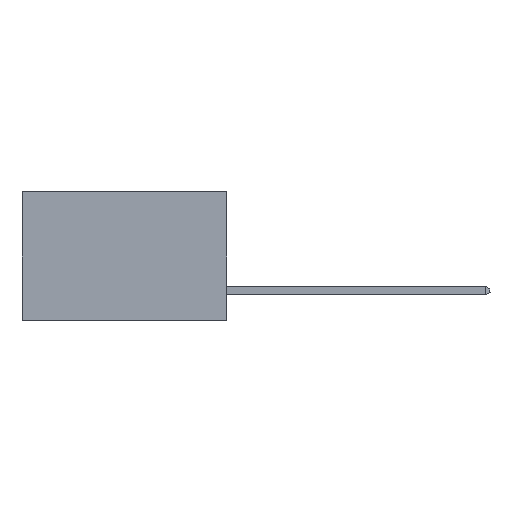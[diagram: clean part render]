
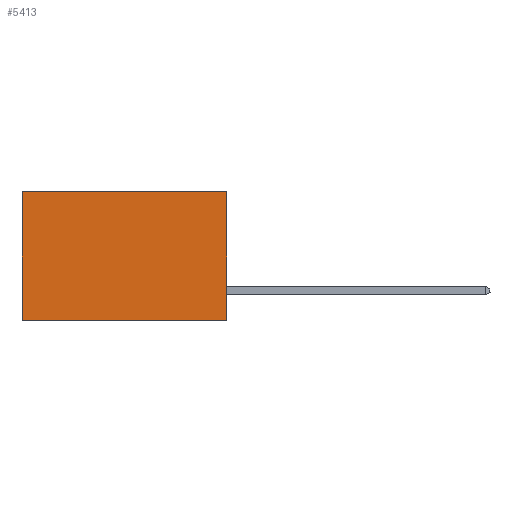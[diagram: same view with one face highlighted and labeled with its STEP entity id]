
A CAD part, left-side view. The second image highlights one B-rep face of the part: STEP entity #5413.
In plain terms, the highlighted planar face has unit normal (-1, 0, 0).
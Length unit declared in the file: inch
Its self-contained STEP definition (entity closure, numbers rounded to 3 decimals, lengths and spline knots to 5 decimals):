
#624 = ORIENTED_EDGE ( 'NONE', *, *, #3565, .F. ) ;
#1215 = CARTESIAN_POINT ( 'NONE',  ( 0.277, 0., -0.37 ) ) ;
#1657 = EDGE_CURVE ( 'NONE', #7869, #6079, #14360, .T. ) ;
#2672 = EDGE_CURVE ( 'NONE', #15554, #18277, #18735, .T. ) ;
#3064 = AXIS2_PLACEMENT_3D ( 'NONE', #20327, #19567, #19518 ) ;
#3565 = EDGE_CURVE ( 'NONE', #6079, #18277, #11058, .T. ) ;
#3865 = LINE ( 'NONE', #8832, #11904 ) ;
#4542 = CARTESIAN_POINT ( 'NONE',  ( 0.277, 0., 0. ) ) ;
#5362 = CARTESIAN_POINT ( 'NONE',  ( 0.277, 0.59, 0. ) ) ;
#5413 = ADVANCED_FACE ( 'NONE', ( #12937 ), #20309, .F. ) ;
#6079 = VERTEX_POINT ( 'NONE', #1215 ) ;
#7869 = VERTEX_POINT ( 'NONE', #4542 ) ;
#8792 = ORIENTED_EDGE ( 'NONE', *, *, #20197, .T. ) ;
#8832 = CARTESIAN_POINT ( 'NONE',  ( 0.277, 0., 0. ) ) ;
#10455 = DIRECTION ( 'NONE',  ( 0., 1., 0. ) ) ;
#10803 = VECTOR ( 'NONE', #17638, 39.37008 ) ;
#11058 = LINE ( 'NONE', #14962, #15305 ) ;
#11408 = CARTESIAN_POINT ( 'NONE',  ( 0.277, 0., -0.37 ) ) ;
#11841 = ORIENTED_EDGE ( 'NONE', *, *, #2672, .T. ) ;
#11904 = VECTOR ( 'NONE', #10455, 39.37008 ) ;
#12937 = FACE_OUTER_BOUND ( 'NONE', #15239, .T. ) ;
#14360 = LINE ( 'NONE', #11408, #19028 ) ;
#14962 = CARTESIAN_POINT ( 'NONE',  ( 0.277, 0., -0.37 ) ) ;
#15239 = EDGE_LOOP ( 'NONE', ( #11841, #624, #18504, #8792 ) ) ;
#15305 = VECTOR ( 'NONE', #17104, 39.37008 ) ;
#15554 = VERTEX_POINT ( 'NONE', #5362 ) ;
#16887 = CARTESIAN_POINT ( 'NONE',  ( 0.277, 0.59, -0.37 ) ) ;
#17104 = DIRECTION ( 'NONE',  ( 0., 1., 0. ) ) ;
#17638 = DIRECTION ( 'NONE',  ( 0., 0., -1. ) ) ;
#17750 = DIRECTION ( 'NONE',  ( 0., 0., -1. ) ) ;
#18277 = VERTEX_POINT ( 'NONE', #16887 ) ;
#18504 = ORIENTED_EDGE ( 'NONE', *, *, #1657, .F. ) ;
#18735 = LINE ( 'NONE', #18819, #10803 ) ;
#18819 = CARTESIAN_POINT ( 'NONE',  ( 0.277, 0.59, -0.37 ) ) ;
#19028 = VECTOR ( 'NONE', #17750, 39.37008 ) ;
#19518 = DIRECTION ( 'NONE',  ( 0., 0., -1. ) ) ;
#19567 = DIRECTION ( 'NONE',  ( 1., 0., 0. ) ) ;
#20197 = EDGE_CURVE ( 'NONE', #7869, #15554, #3865, .T. ) ;
#20309 = PLANE ( 'NONE',  #3064 ) ;
#20327 = CARTESIAN_POINT ( 'NONE',  ( 0.277, 0., -0.37 ) ) ;
